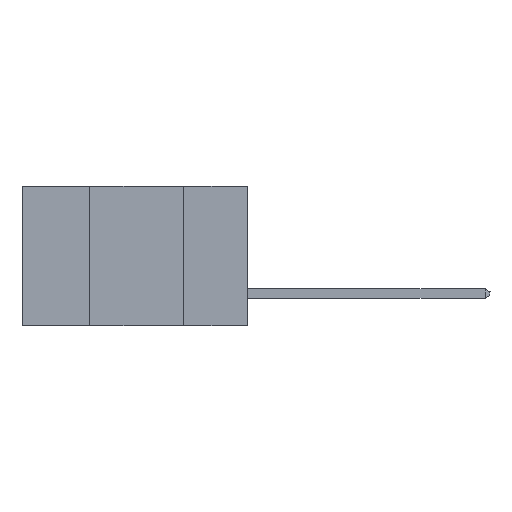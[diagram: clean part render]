
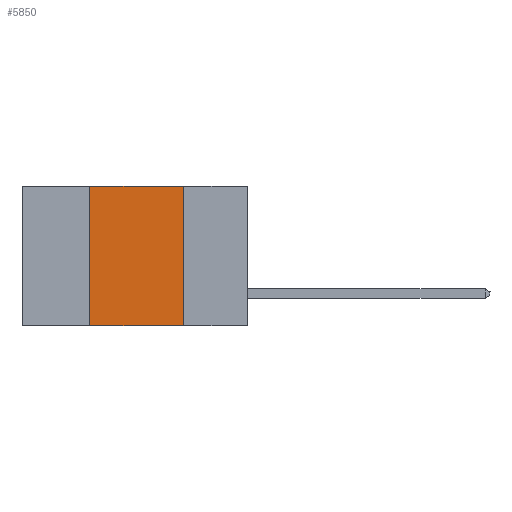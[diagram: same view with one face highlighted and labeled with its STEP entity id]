
A CAD part, left-side view. The second image highlights one B-rep face of the part: STEP entity #5850.
In plain terms, the highlighted planar face has unit normal (-1, 0, 0).
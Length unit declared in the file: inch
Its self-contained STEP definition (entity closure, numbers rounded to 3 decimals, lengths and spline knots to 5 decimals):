
#1069 = LINE ( 'NONE', #4414, #4478 ) ;
#1280 = EDGE_CURVE ( 'NONE', #4316, #10132, #8471, .T. ) ;
#1507 = LINE ( 'NONE', #9230, #3987 ) ;
#1793 = ORIENTED_EDGE ( 'NONE', *, *, #1280, .F. ) ;
#2256 = AXIS2_PLACEMENT_3D ( 'NONE', #9241, #6019, #10242 ) ;
#2511 = CARTESIAN_POINT ( 'NONE',  ( 0., 0.17, -0.37 ) ) ;
#2533 = CARTESIAN_POINT ( 'NONE',  ( 0., 0.42, -0.37 ) ) ;
#3316 = ORIENTED_EDGE ( 'NONE', *, *, #10752, .F. ) ;
#3352 = VERTEX_POINT ( 'NONE', #2533 ) ;
#3701 = VERTEX_POINT ( 'NONE', #2511 ) ;
#3783 = CARTESIAN_POINT ( 'NONE',  ( 0., 0.42, 0. ) ) ;
#3987 = VECTOR ( 'NONE', #5737, 39.37008 ) ;
#4258 = DIRECTION ( 'NONE',  ( 0., -1., 0. ) ) ;
#4316 = VERTEX_POINT ( 'NONE', #3783 ) ;
#4414 = CARTESIAN_POINT ( 'NONE',  ( 0., 0.17, -0.37 ) ) ;
#4478 = VECTOR ( 'NONE', #9615, 39.37008 ) ;
#4966 = ORIENTED_EDGE ( 'NONE', *, *, #7709, .F. ) ;
#5023 = FACE_OUTER_BOUND ( 'NONE', #5785, .T. ) ;
#5173 = VECTOR ( 'NONE', #8293, 39.37008 ) ;
#5737 = DIRECTION ( 'NONE',  ( 0., 0., 1. ) ) ;
#5785 = EDGE_LOOP ( 'NONE', ( #4966, #1793, #3316, #8161 ) ) ;
#5850 = ADVANCED_FACE ( 'NONE', ( #5023 ), #5855, .F. ) ;
#5855 = PLANE ( 'NONE',  #2256 ) ;
#6019 = DIRECTION ( 'NONE',  ( 1., 0., 0. ) ) ;
#6996 = CARTESIAN_POINT ( 'NONE',  ( 0., 0.17, 0. ) ) ;
#7407 = EDGE_CURVE ( 'NONE', #3352, #3701, #9058, .T. ) ;
#7709 = EDGE_CURVE ( 'NONE', #10132, #3701, #1069, .T. ) ;
#8161 = ORIENTED_EDGE ( 'NONE', *, *, #7407, .T. ) ;
#8293 = DIRECTION ( 'NONE',  ( 0., -1., 0. ) ) ;
#8471 = LINE ( 'NONE', #8631, #9877 ) ;
#8631 = CARTESIAN_POINT ( 'NONE',  ( 0., 0.6, 0. ) ) ;
#9058 = LINE ( 'NONE', #10677, #5173 ) ;
#9230 = CARTESIAN_POINT ( 'NONE',  ( 0., 0.42, -0.37 ) ) ;
#9241 = CARTESIAN_POINT ( 'NONE',  ( 0., 0.6, 0. ) ) ;
#9615 = DIRECTION ( 'NONE',  ( 0., 0., -1. ) ) ;
#9877 = VECTOR ( 'NONE', #4258, 39.37008 ) ;
#10132 = VERTEX_POINT ( 'NONE', #6996 ) ;
#10242 = DIRECTION ( 'NONE',  ( 0., 0., -1. ) ) ;
#10677 = CARTESIAN_POINT ( 'NONE',  ( 0., 0.6, -0.37 ) ) ;
#10752 = EDGE_CURVE ( 'NONE', #3352, #4316, #1507, .T. ) ;
